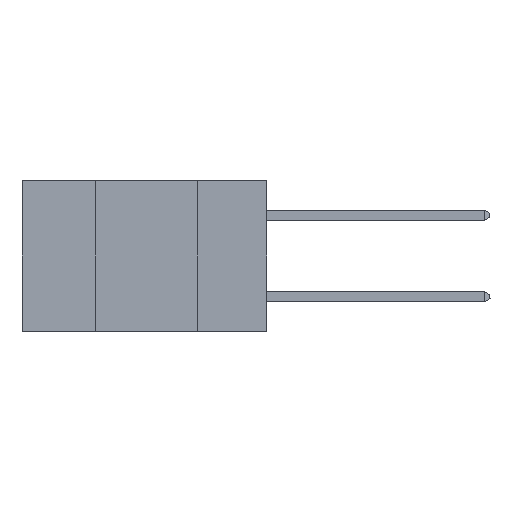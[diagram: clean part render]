
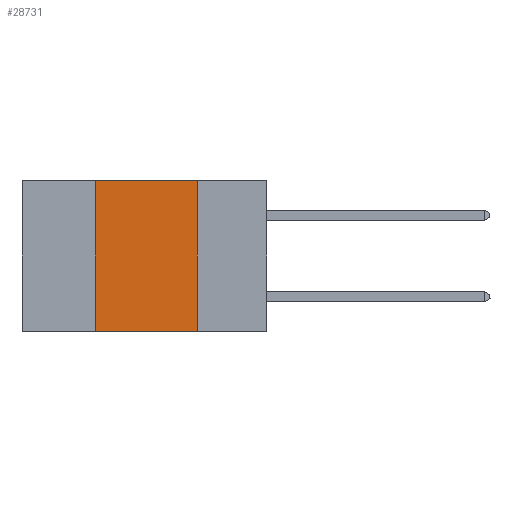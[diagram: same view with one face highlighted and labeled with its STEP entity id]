
A CAD part, left-side view. The second image highlights one B-rep face of the part: STEP entity #28731.
In plain terms, the highlighted planar face has unit normal (-1, 0, 0).
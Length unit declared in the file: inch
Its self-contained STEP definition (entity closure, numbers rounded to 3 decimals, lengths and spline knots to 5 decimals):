
#770 = VERTEX_POINT ( 'NONE', #1252 ) ;
#859 = VERTEX_POINT ( 'NONE', #15795 ) ;
#1252 = CARTESIAN_POINT ( 'NONE',  ( 0., 0.42, -0.37 ) ) ;
#2195 = DIRECTION ( 'NONE',  ( 0., 0., -1. ) ) ;
#2407 = CARTESIAN_POINT ( 'NONE',  ( 0., 0.17, 0. ) ) ;
#3411 = CARTESIAN_POINT ( 'NONE',  ( 0., 0.6, -0.37 ) ) ;
#3812 = VECTOR ( 'NONE', #2195, 39.37008 ) ;
#4213 = EDGE_CURVE ( 'NONE', #23286, #859, #21335, .T. ) ;
#5159 = EDGE_LOOP ( 'NONE', ( #15962, #12819, #15163, #29332 ) ) ;
#6460 = EDGE_CURVE ( 'NONE', #770, #31029, #28952, .T. ) ;
#8175 = VECTOR ( 'NONE', #27852, 39.37008 ) ;
#8918 = CARTESIAN_POINT ( 'NONE',  ( 0., 0.42, 0. ) ) ;
#10623 = VECTOR ( 'NONE', #28334, 39.37008 ) ;
#10632 = AXIS2_PLACEMENT_3D ( 'NONE', #29134, #14670, #19520 ) ;
#10983 = LINE ( 'NONE', #2407, #3812 ) ;
#11682 = CARTESIAN_POINT ( 'NONE',  ( 0., 0.17, -0.37 ) ) ;
#12130 = LINE ( 'NONE', #8918, #10623 ) ;
#12179 = EDGE_CURVE ( 'NONE', #859, #31029, #10983, .T. ) ;
#12819 = ORIENTED_EDGE ( 'NONE', *, *, #4213, .F. ) ;
#14670 = DIRECTION ( 'NONE',  ( 1., 0., 0. ) ) ;
#15163 = ORIENTED_EDGE ( 'NONE', *, *, #27723, .F. ) ;
#15795 = CARTESIAN_POINT ( 'NONE',  ( 0., 0.17, 0. ) ) ;
#15962 = ORIENTED_EDGE ( 'NONE', *, *, #12179, .F. ) ;
#17876 = DIRECTION ( 'NONE',  ( 0., -1., 0. ) ) ;
#19520 = DIRECTION ( 'NONE',  ( 0., 0., -1. ) ) ;
#19768 = CARTESIAN_POINT ( 'NONE',  ( 0., 0.42, 0. ) ) ;
#21335 = LINE ( 'NONE', #22520, #31095 ) ;
#22520 = CARTESIAN_POINT ( 'NONE',  ( 0., 0.6, 0. ) ) ;
#23286 = VERTEX_POINT ( 'NONE', #19768 ) ;
#24681 = PLANE ( 'NONE',  #10632 ) ;
#27723 = EDGE_CURVE ( 'NONE', #770, #23286, #12130, .T. ) ;
#27852 = DIRECTION ( 'NONE',  ( 0., -1., 0. ) ) ;
#28334 = DIRECTION ( 'NONE',  ( 0., 0., 1. ) ) ;
#28731 = ADVANCED_FACE ( 'NONE', ( #29075 ), #24681, .F. ) ;
#28952 = LINE ( 'NONE', #3411, #8175 ) ;
#29075 = FACE_OUTER_BOUND ( 'NONE', #5159, .T. ) ;
#29134 = CARTESIAN_POINT ( 'NONE',  ( 0., 0.6, 0. ) ) ;
#29332 = ORIENTED_EDGE ( 'NONE', *, *, #6460, .T. ) ;
#31029 = VERTEX_POINT ( 'NONE', #11682 ) ;
#31095 = VECTOR ( 'NONE', #17876, 39.37008 ) ;
